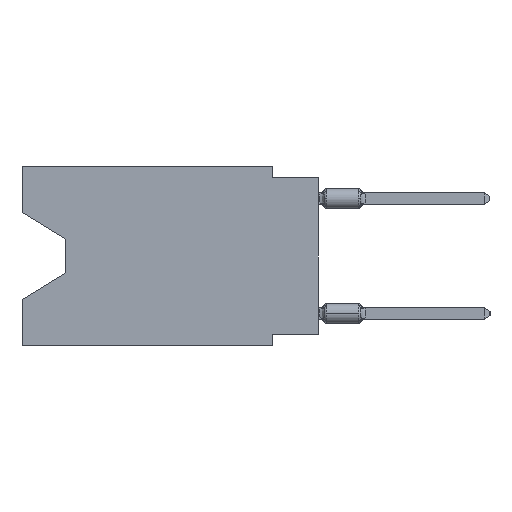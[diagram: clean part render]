
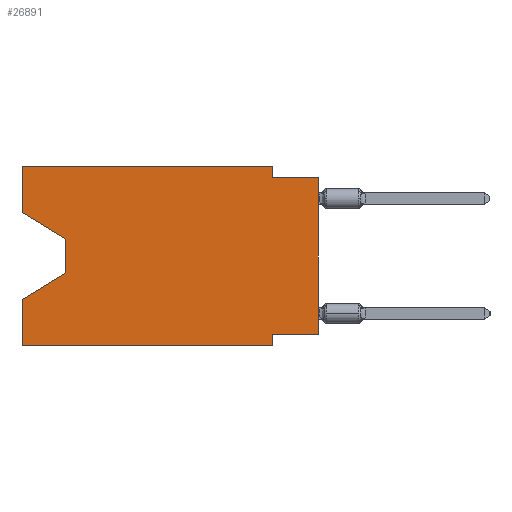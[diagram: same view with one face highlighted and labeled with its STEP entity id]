
A CAD part, left-side view. The second image highlights one B-rep face of the part: STEP entity #26891.
In plain terms, the highlighted planar face has unit normal (-1, 0, 0).
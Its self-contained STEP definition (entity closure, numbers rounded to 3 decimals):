
#31 = CARTESIAN_POINT ( 'NONE',  ( 0., 0., -0.635 ) ) ;
#1148 = LINE ( 'NONE', #53394, #48686 ) ;
#1915 = CARTESIAN_POINT ( 'NONE',  ( 0., 16.383, 0. ) ) ;
#4110 = ORIENTED_EDGE ( 'NONE', *, *, #10140, .F. ) ;
#4986 = ORIENTED_EDGE ( 'NONE', *, *, #46562, .F. ) ;
#6708 = CARTESIAN_POINT ( 'NONE',  ( 0., 16.383, -2.546 ) ) ;
#6918 = EDGE_CURVE ( 'NONE', #21753, #55635, #11592, .T. ) ;
#7144 = CARTESIAN_POINT ( 'NONE',  ( 0., 13.97, -4.013 ) ) ;
#8994 = DIRECTION ( 'NONE',  ( 0., -1., 0. ) ) ;
#9144 = ORIENTED_EDGE ( 'NONE', *, *, #6918, .F. ) ;
#10140 = EDGE_CURVE ( 'NONE', #21744, #21753, #50165, .T. ) ;
#10757 = CARTESIAN_POINT ( 'NONE',  ( 0., 0., -9.271 ) ) ;
#11000 = LINE ( 'NONE', #23565, #14353 ) ;
#11163 = VECTOR ( 'NONE', #37317, 1000. ) ;
#11592 = LINE ( 'NONE', #29570, #25985 ) ;
#11717 = ORIENTED_EDGE ( 'NONE', *, *, #17682, .T. ) ;
#12003 = VECTOR ( 'NONE', #30672, 1000. ) ;
#12900 = ORIENTED_EDGE ( 'NONE', *, *, #19039, .T. ) ;
#13993 = DIRECTION ( 'NONE',  ( 0., -1., 0. ) ) ;
#14353 = VECTOR ( 'NONE', #19289, 1000. ) ;
#15310 = VERTEX_POINT ( 'NONE', #51715 ) ;
#15335 = LINE ( 'NONE', #1915, #11163 ) ;
#15342 = LINE ( 'NONE', #32756, #48604 ) ;
#16019 = PLANE ( 'NONE',  #41692 ) ;
#16288 = EDGE_CURVE ( 'NONE', #50903, #40659, #32702, .T. ) ;
#16577 = DIRECTION ( 'NONE',  ( 1., 0., 0. ) ) ;
#16973 = ORIENTED_EDGE ( 'NONE', *, *, #16288, .T. ) ;
#17271 = LINE ( 'NONE', #48123, #53102 ) ;
#17682 = EDGE_CURVE ( 'NONE', #26120, #38514, #18492, .T. ) ;
#17686 = CARTESIAN_POINT ( 'NONE',  ( 0., 2.54, 0. ) ) ;
#17814 = EDGE_CURVE ( 'NONE', #47436, #20296, #15335, .T. ) ;
#18492 = LINE ( 'NONE', #44198, #47618 ) ;
#18658 = CARTESIAN_POINT ( 'NONE',  ( 0., 16.383, 0. ) ) ;
#19039 = EDGE_CURVE ( 'NONE', #15310, #55635, #1148, .T. ) ;
#19289 = DIRECTION ( 'NONE',  ( 0., 0., 1. ) ) ;
#19911 = EDGE_LOOP ( 'NONE', ( #16973, #49307, #11717, #4986, #12900, #9144, #4110, #30124, #29612, #37422, #45442, #29006 ) ) ;
#20296 = VERTEX_POINT ( 'NONE', #49682 ) ;
#20954 = CARTESIAN_POINT ( 'NONE',  ( 0., 16.383, -7.36 ) ) ;
#21111 = EDGE_CURVE ( 'NONE', #40659, #26120, #15342, .T. ) ;
#21510 = VECTOR ( 'NONE', #53511, 1000. ) ;
#21744 = VERTEX_POINT ( 'NONE', #35710 ) ;
#21753 = VERTEX_POINT ( 'NONE', #40277 ) ;
#22657 = CARTESIAN_POINT ( 'NONE',  ( 0., 2.54, -0.635 ) ) ;
#23565 = CARTESIAN_POINT ( 'NONE',  ( 0., 0., 0. ) ) ;
#25370 = EDGE_CURVE ( 'NONE', #50903, #47436, #36097, .T. ) ;
#25985 = VECTOR ( 'NONE', #46991, 1000. ) ;
#26120 = VERTEX_POINT ( 'NONE', #35401 ) ;
#26183 = EDGE_CURVE ( 'NONE', #20296, #38678, #39394, .T. ) ;
#26891 = ADVANCED_FACE ( 'NONE', ( #29158 ), #16019, .F. ) ;
#27087 = VERTEX_POINT ( 'NONE', #31 ) ;
#27245 = CARTESIAN_POINT ( 'NONE',  ( 0., 16.383, 0. ) ) ;
#29006 = ORIENTED_EDGE ( 'NONE', *, *, #25370, .F. ) ;
#29158 = FACE_OUTER_BOUND ( 'NONE', #19911, .T. ) ;
#29570 = CARTESIAN_POINT ( 'NONE',  ( 0., 2.54, -9.906 ) ) ;
#29612 = ORIENTED_EDGE ( 'NONE', *, *, #49090, .F. ) ;
#30124 = ORIENTED_EDGE ( 'NONE', *, *, #39680, .T. ) ;
#30672 = DIRECTION ( 'NONE',  ( 0., 0., 1. ) ) ;
#30780 = DIRECTION ( 'NONE',  ( 0., 0.855, -0.519 ) ) ;
#31862 = CARTESIAN_POINT ( 'NONE',  ( 0., 16.383, 0. ) ) ;
#32167 = DIRECTION ( 'NONE',  ( 0., 1., 0. ) ) ;
#32702 = LINE ( 'NONE', #6708, #34903 ) ;
#32756 = CARTESIAN_POINT ( 'NONE',  ( 0., 13.97, -4.013 ) ) ;
#34903 = VECTOR ( 'NONE', #50128, 1000. ) ;
#35114 = DIRECTION ( 'NONE',  ( 0., 0., -1. ) ) ;
#35401 = CARTESIAN_POINT ( 'NONE',  ( 0., 13.97, -5.893 ) ) ;
#35710 = CARTESIAN_POINT ( 'NONE',  ( 0., 0., -9.271 ) ) ;
#36097 = LINE ( 'NONE', #27245, #21510 ) ;
#37317 = DIRECTION ( 'NONE',  ( 0., -1., 0. ) ) ;
#37422 = ORIENTED_EDGE ( 'NONE', *, *, #26183, .F. ) ;
#38514 = VERTEX_POINT ( 'NONE', #20954 ) ;
#38675 = LINE ( 'NONE', #18658, #12003 ) ;
#38678 = VERTEX_POINT ( 'NONE', #22657 ) ;
#39394 = LINE ( 'NONE', #17686, #44404 ) ;
#39680 = EDGE_CURVE ( 'NONE', #21744, #27087, #11000, .T. ) ;
#40277 = CARTESIAN_POINT ( 'NONE',  ( 0., 2.54, -9.271 ) ) ;
#40659 = VERTEX_POINT ( 'NONE', #7144 ) ;
#41692 = AXIS2_PLACEMENT_3D ( 'NONE', #47147, #16577, #51418 ) ;
#41838 = VECTOR ( 'NONE', #32167, 1000. ) ;
#43414 = CARTESIAN_POINT ( 'NONE',  ( 0., 16.383, -2.546 ) ) ;
#44198 = CARTESIAN_POINT ( 'NONE',  ( 0., 13.97, -5.893 ) ) ;
#44404 = VECTOR ( 'NONE', #35114, 1000. ) ;
#45442 = ORIENTED_EDGE ( 'NONE', *, *, #17814, .F. ) ;
#46562 = EDGE_CURVE ( 'NONE', #15310, #38514, #38675, .T. ) ;
#46991 = DIRECTION ( 'NONE',  ( 0., 0., -1. ) ) ;
#47147 = CARTESIAN_POINT ( 'NONE',  ( 0., 16.383, 0. ) ) ;
#47436 = VERTEX_POINT ( 'NONE', #31862 ) ;
#47531 = CARTESIAN_POINT ( 'NONE',  ( 0., 2.54, -9.906 ) ) ;
#47618 = VECTOR ( 'NONE', #30780, 1000. ) ;
#48123 = CARTESIAN_POINT ( 'NONE',  ( 0., 0., -0.635 ) ) ;
#48604 = VECTOR ( 'NONE', #50181, 1000. ) ;
#48686 = VECTOR ( 'NONE', #13993, 1000. ) ;
#49090 = EDGE_CURVE ( 'NONE', #38678, #27087, #17271, .T. ) ;
#49307 = ORIENTED_EDGE ( 'NONE', *, *, #21111, .T. ) ;
#49682 = CARTESIAN_POINT ( 'NONE',  ( 0., 2.54, 0. ) ) ;
#50128 = DIRECTION ( 'NONE',  ( 0., -0.855, -0.519 ) ) ;
#50165 = LINE ( 'NONE', #10757, #41838 ) ;
#50181 = DIRECTION ( 'NONE',  ( 0., 0., -1. ) ) ;
#50903 = VERTEX_POINT ( 'NONE', #43414 ) ;
#51418 = DIRECTION ( 'NONE',  ( 0., 0., -1. ) ) ;
#51715 = CARTESIAN_POINT ( 'NONE',  ( 0., 16.383, -9.906 ) ) ;
#53102 = VECTOR ( 'NONE', #8994, 1000. ) ;
#53394 = CARTESIAN_POINT ( 'NONE',  ( 0., 16.383, -9.906 ) ) ;
#53511 = DIRECTION ( 'NONE',  ( 0., 0., 1. ) ) ;
#55635 = VERTEX_POINT ( 'NONE', #47531 ) ;
